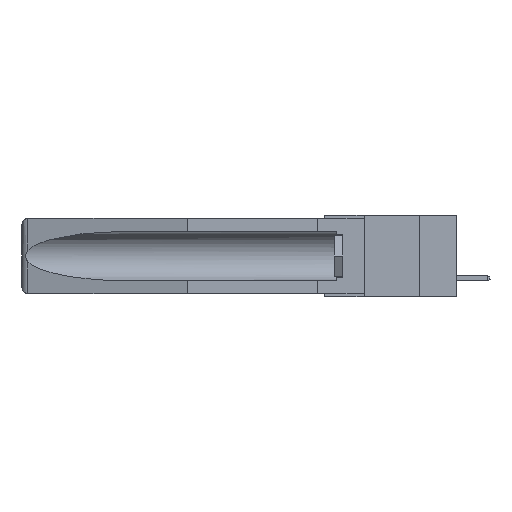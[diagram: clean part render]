
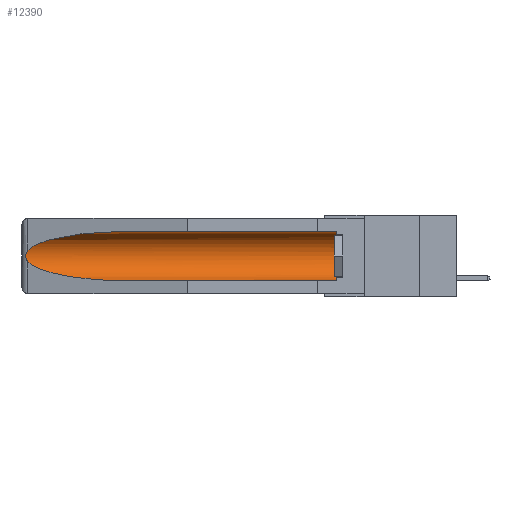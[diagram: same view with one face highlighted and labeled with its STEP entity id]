
A CAD part, left-side view. The second image highlights one B-rep face of the part: STEP entity #12390.
In plain terms, the highlighted cylindrical face has radius 2.857 mm (diameter 5.715 mm), a partial arc.
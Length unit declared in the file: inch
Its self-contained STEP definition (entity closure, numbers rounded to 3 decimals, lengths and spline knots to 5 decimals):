
#166 =( BOUNDED_CURVE ( )  B_SPLINE_CURVE ( 3, ( #3120, #21470, #13077, #23276 ),
 .UNSPECIFIED., .F., .F. ) 
 B_SPLINE_CURVE_WITH_KNOTS ( ( 4, 4 ),
 ( 4.71239, 6.08839 ),
 .UNSPECIFIED. ) 
 CURVE ( )  GEOMETRIC_REPRESENTATION_ITEM ( )  RATIONAL_B_SPLINE_CURVE ( ( 1., 0.848, 0.848, 1. ) ) 
 REPRESENTATION_ITEM ( '' )  );
#246 = VERTEX_POINT ( 'NONE', #11292 ) ;
#1853 = ORIENTED_EDGE ( 'NONE', *, *, #19871, .T. ) ;
#2958 = AXIS2_PLACEMENT_3D ( 'NONE', #23615, #19494, #17415 ) ;
#3120 = CARTESIAN_POINT ( 'NONE',  ( 0.155, 1.07973, -0.059 ) ) ;
#3229 = CARTESIAN_POINT ( 'NONE',  ( 0.26597, 1.52961, -0.15275 ) ) ;
#3408 = CARTESIAN_POINT ( 'NONE',  ( 0.2673, 1.5327, -0.16383 ) ) ;
#3607 = B_SPLINE_CURVE_WITH_KNOTS ( 'NONE', 3,
 ( #19719, #3229, #21670, #3408, #7484, #23663, #17374, #5206, #17560, #23474 ),
 .UNSPECIFIED., .F., .F.,
 ( 4, 2, 2, 2, 4 ),
 ( 0., 0.00029, 0.00058, 0.00087, 0.00117 ),
 .UNSPECIFIED. ) ;
#5206 = CARTESIAN_POINT ( 'NONE',  ( 0.26655, 1.53094, -0.18657 ) ) ;
#5997 = DIRECTION ( 'NONE',  ( 0., 1., 0. ) ) ;
#6056 = VERTEX_POINT ( 'NONE', #15723 ) ;
#6281 = DIRECTION ( 'NONE',  ( 0., -1., 0. ) ) ;
#7484 = CARTESIAN_POINT ( 'NONE',  ( 0.2675, 1.53308, -0.16763 ) ) ;
#8336 = VECTOR ( 'NONE', #17279, 39.37008 ) ;
#10155 = CARTESIAN_POINT ( 'NONE',  ( 0.155, -0.30754, -0.059 ) ) ;
#10193 = EDGE_LOOP ( 'NONE', ( #1853, #20810, #11364, #12055, #22449, #19048 ) ) ;
#10349 = DIRECTION ( 'NONE',  ( 0., 0., 1. ) ) ;
#11136 = CIRCLE ( 'NONE', #19726, 0.1125 ) ;
#11292 = CARTESIAN_POINT ( 'NONE',  ( 0.26537, 1.52718, -0.19328 ) ) ;
#11364 = ORIENTED_EDGE ( 'NONE', *, *, #24908, .T. ) ;
#12055 = ORIENTED_EDGE ( 'NONE', *, *, #23640, .F. ) ;
#12390 = ADVANCED_FACE ( 'NONE', ( #18655 ), #19289, .F. ) ;
#13034 =( BOUNDED_CURVE ( )  B_SPLINE_CURVE ( 3, ( #21328, #17382, #13190, #13379 ),
 .UNSPECIFIED., .F., .F. ) 
 B_SPLINE_CURVE_WITH_KNOTS ( ( 4, 4 ),
 ( 0.1948, 1.5708 ),
 .UNSPECIFIED. ) 
 CURVE ( )  GEOMETRIC_REPRESENTATION_ITEM ( )  RATIONAL_B_SPLINE_CURVE ( ( 1., 0.848, 0.848, 1. ) ) 
 REPRESENTATION_ITEM ( '' )  );
#13077 = CARTESIAN_POINT ( 'NONE',  ( 0.25451, 1.48313, -0.09465 ) ) ;
#13190 = CARTESIAN_POINT ( 'NONE',  ( 0.21114, 1.30732, -0.284 ) ) ;
#13379 = CARTESIAN_POINT ( 'NONE',  ( 0.155, 1.07973, -0.284 ) ) ;
#13732 = CARTESIAN_POINT ( 'NONE',  ( 0.155, 1.07973, -0.284 ) ) ;
#13814 = VERTEX_POINT ( 'NONE', #26093 ) ;
#14396 = CARTESIAN_POINT ( 'NONE',  ( 0.155, 0.126, -0.1715 ) ) ;
#14708 = CARTESIAN_POINT ( 'NONE',  ( 0.155, 0.126, -0.059 ) ) ;
#15244 = CARTESIAN_POINT ( 'NONE',  ( 0.155, -0.30754, -0.284 ) ) ;
#15313 = EDGE_CURVE ( 'NONE', #23076, #246, #3607, .T. ) ;
#15723 = CARTESIAN_POINT ( 'NONE',  ( 0.155, 1.07973, -0.059 ) ) ;
#17279 = DIRECTION ( 'NONE',  ( 0., 1., 0. ) ) ;
#17374 = CARTESIAN_POINT ( 'NONE',  ( 0.2673, 1.53269, -0.17917 ) ) ;
#17382 = CARTESIAN_POINT ( 'NONE',  ( 0.25451, 1.48313, -0.24835 ) ) ;
#17415 = DIRECTION ( 'NONE',  ( 0., 0., 1. ) ) ;
#17560 = CARTESIAN_POINT ( 'NONE',  ( 0.26597, 1.5296, -0.19026 ) ) ;
#18510 = LINE ( 'NONE', #10155, #22030 ) ;
#18655 = FACE_OUTER_BOUND ( 'NONE', #10193, .T. ) ;
#19048 = ORIENTED_EDGE ( 'NONE', *, *, #20499, .T. ) ;
#19289 = CYLINDRICAL_SURFACE ( 'NONE', #2958, 0.1125 ) ;
#19494 = DIRECTION ( 'NONE',  ( 0., 1., 0. ) ) ;
#19719 = CARTESIAN_POINT ( 'NONE',  ( 0.26537, 1.52718, -0.14972 ) ) ;
#19726 = AXIS2_PLACEMENT_3D ( 'NONE', #14396, #6281, #10349 ) ;
#19871 = EDGE_CURVE ( 'NONE', #6056, #23076, #166, .T. ) ;
#20499 = EDGE_CURVE ( 'NONE', #21866, #6056, #18510, .T. ) ;
#20805 = LINE ( 'NONE', #15244, #8336 ) ;
#20810 = ORIENTED_EDGE ( 'NONE', *, *, #15313, .T. ) ;
#21328 = CARTESIAN_POINT ( 'NONE',  ( 0.26537, 1.52718, -0.19328 ) ) ;
#21470 = CARTESIAN_POINT ( 'NONE',  ( 0.21114, 1.30732, -0.059 ) ) ;
#21600 = VERTEX_POINT ( 'NONE', #13732 ) ;
#21670 = CARTESIAN_POINT ( 'NONE',  ( 0.26654, 1.53092, -0.15636 ) ) ;
#21866 = VERTEX_POINT ( 'NONE', #14708 ) ;
#22030 = VECTOR ( 'NONE', #5997, 39.37008 ) ;
#22449 = ORIENTED_EDGE ( 'NONE', *, *, #24700, .T. ) ;
#23076 = VERTEX_POINT ( 'NONE', #24141 ) ;
#23276 = CARTESIAN_POINT ( 'NONE',  ( 0.26537, 1.52718, -0.14972 ) ) ;
#23474 = CARTESIAN_POINT ( 'NONE',  ( 0.26537, 1.52718, -0.19328 ) ) ;
#23615 = CARTESIAN_POINT ( 'NONE',  ( 0.155, -0.30754, -0.1715 ) ) ;
#23640 = EDGE_CURVE ( 'NONE', #13814, #21600, #20805, .T. ) ;
#23663 = CARTESIAN_POINT ( 'NONE',  ( 0.2675, 1.53308, -0.17534 ) ) ;
#24141 = CARTESIAN_POINT ( 'NONE',  ( 0.26537, 1.52718, -0.14972 ) ) ;
#24700 = EDGE_CURVE ( 'NONE', #13814, #21866, #11136, .T. ) ;
#24908 = EDGE_CURVE ( 'NONE', #246, #21600, #13034, .T. ) ;
#26093 = CARTESIAN_POINT ( 'NONE',  ( 0.155, 0.126, -0.284 ) ) ;
